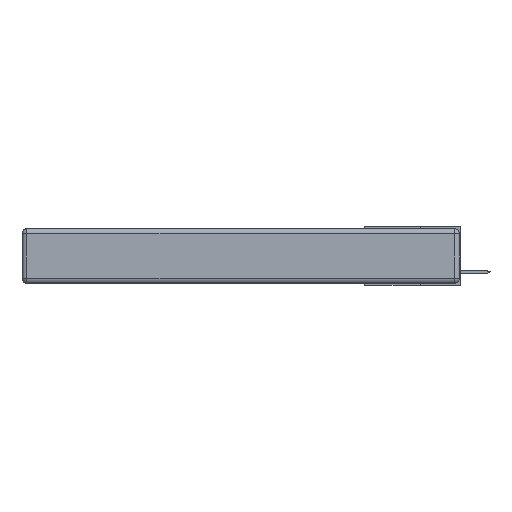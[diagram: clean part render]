
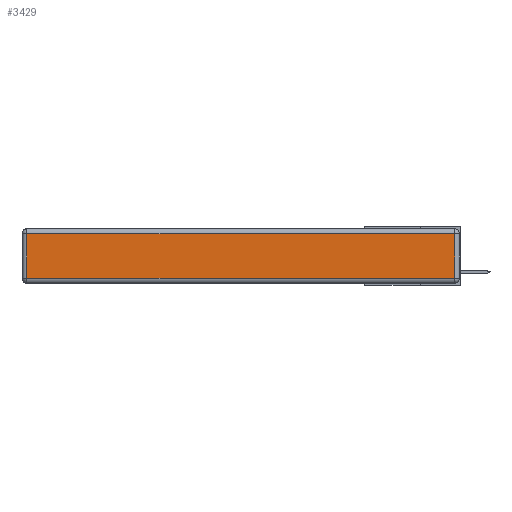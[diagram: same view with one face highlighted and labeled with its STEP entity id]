
A CAD part, left-side view. The second image highlights one B-rep face of the part: STEP entity #3429.
In plain terms, the highlighted planar face has unit normal (-1, 0, 0).
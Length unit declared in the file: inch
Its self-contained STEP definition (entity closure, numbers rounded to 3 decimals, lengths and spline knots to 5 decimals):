
#227 = VECTOR ( 'NONE', #5790, 39.37008 ) ;
#392 = EDGE_CURVE ( 'NONE', #10875, #14340, #21978, .T. ) ;
#678 = CARTESIAN_POINT ( 'NONE',  ( 0., 2.72, -0.343 ) ) ;
#812 = DIRECTION ( 'NONE',  ( 0., 0., -1. ) ) ;
#870 = VECTOR ( 'NONE', #16745, 39.37008 ) ;
#932 = ORIENTED_EDGE ( 'NONE', *, *, #1993, .T. ) ;
#1394 = LINE ( 'NONE', #19494, #9682 ) ;
#1634 = DIRECTION ( 'NONE',  ( -1., 0., 0. ) ) ;
#1993 = EDGE_CURVE ( 'NONE', #3984, #10875, #6281, .T. ) ;
#2994 = DIRECTION ( 'NONE',  ( 0., 1., 0. ) ) ;
#3429 = ADVANCED_FACE ( 'NONE', ( #21377 ), #5445, .T. ) ;
#3984 = VERTEX_POINT ( 'NONE', #20607 ) ;
#5445 = PLANE ( 'NONE',  #12699 ) ;
#5790 = DIRECTION ( 'NONE',  ( 0., 0., 1. ) ) ;
#6151 = CARTESIAN_POINT ( 'NONE',  ( 0., 0.03, -0.03 ) ) ;
#6281 = LINE ( 'NONE', #13108, #870 ) ;
#6366 = EDGE_LOOP ( 'NONE', ( #932, #14705, #14571, #19184 ) ) ;
#7683 = CARTESIAN_POINT ( 'NONE',  ( 0., 0.03, -0.343 ) ) ;
#9682 = VECTOR ( 'NONE', #2994, 39.37008 ) ;
#10741 = DIRECTION ( 'NONE',  ( 0., 0., 1. ) ) ;
#10875 = VERTEX_POINT ( 'NONE', #15705 ) ;
#12699 = AXIS2_PLACEMENT_3D ( 'NONE', #17961, #1634, #10741 ) ;
#13108 = CARTESIAN_POINT ( 'NONE',  ( 0., 0., -0.313 ) ) ;
#14340 = VERTEX_POINT ( 'NONE', #6151 ) ;
#14571 = ORIENTED_EDGE ( 'NONE', *, *, #17546, .T. ) ;
#14705 = ORIENTED_EDGE ( 'NONE', *, *, #392, .T. ) ;
#15299 = LINE ( 'NONE', #678, #18438 ) ;
#15705 = CARTESIAN_POINT ( 'NONE',  ( 0., 0.03, -0.313 ) ) ;
#16745 = DIRECTION ( 'NONE',  ( 0., -1., 0. ) ) ;
#17546 = EDGE_CURVE ( 'NONE', #14340, #22424, #1394, .T. ) ;
#17961 = CARTESIAN_POINT ( 'NONE',  ( 0., 0., -0.343 ) ) ;
#18438 = VECTOR ( 'NONE', #812, 39.37008 ) ;
#19184 = ORIENTED_EDGE ( 'NONE', *, *, #20588, .T. ) ;
#19192 = CARTESIAN_POINT ( 'NONE',  ( 0., 2.72, -0.03 ) ) ;
#19494 = CARTESIAN_POINT ( 'NONE',  ( 0., 2.75, -0.03 ) ) ;
#20588 = EDGE_CURVE ( 'NONE', #22424, #3984, #15299, .T. ) ;
#20607 = CARTESIAN_POINT ( 'NONE',  ( 0., 2.72, -0.313 ) ) ;
#21377 = FACE_OUTER_BOUND ( 'NONE', #6366, .T. ) ;
#21978 = LINE ( 'NONE', #7683, #227 ) ;
#22424 = VERTEX_POINT ( 'NONE', #19192 ) ;
